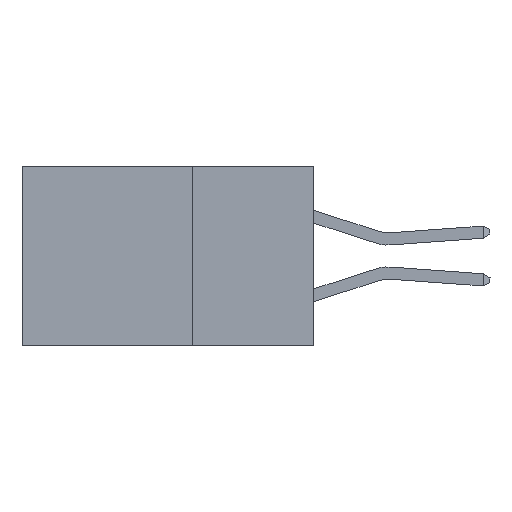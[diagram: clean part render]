
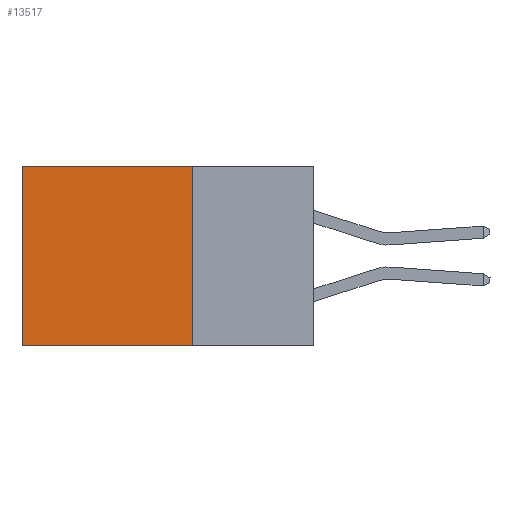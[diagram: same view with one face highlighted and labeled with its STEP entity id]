
A CAD part, left-side view. The second image highlights one B-rep face of the part: STEP entity #13517.
In plain terms, the highlighted planar face has unit normal (-1, 0, 0).
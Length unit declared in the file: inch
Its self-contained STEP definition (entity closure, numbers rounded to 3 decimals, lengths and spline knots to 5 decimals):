
#1093 = AXIS2_PLACEMENT_3D ( 'NONE', #13109, #39738, #36252 ) ;
#1731 = VERTEX_POINT ( 'NONE', #4457 ) ;
#2899 = PLANE ( 'NONE',  #1093 ) ;
#4457 = CARTESIAN_POINT ( 'NONE',  ( 0.2875, 0.25, 0. ) ) ;
#6165 = VERTEX_POINT ( 'NONE', #38595 ) ;
#7071 = ORIENTED_EDGE ( 'NONE', *, *, #35194, .F. ) ;
#8309 = ORIENTED_EDGE ( 'NONE', *, *, #19649, .T. ) ;
#9056 = VECTOR ( 'NONE', #27828, 39.37008 ) ;
#9360 = VERTEX_POINT ( 'NONE', #19835 ) ;
#10572 = CARTESIAN_POINT ( 'NONE',  ( 0.2875, 0.25, -0.37 ) ) ;
#13109 = CARTESIAN_POINT ( 'NONE',  ( 0.2875, 0.25, 0. ) ) ;
#13501 = EDGE_CURVE ( 'NONE', #6165, #21395, #30585, .T. ) ;
#13517 = ADVANCED_FACE ( 'NONE', ( #21168 ), #2899, .F. ) ;
#15517 = EDGE_CURVE ( 'NONE', #1731, #9360, #16249, .T. ) ;
#16249 = LINE ( 'NONE', #28277, #21497 ) ;
#19649 = EDGE_CURVE ( 'NONE', #1731, #6165, #43074, .T. ) ;
#19835 = CARTESIAN_POINT ( 'NONE',  ( 0.2875, 0.25, -0.37 ) ) ;
#21168 = FACE_OUTER_BOUND ( 'NONE', #21216, .T. ) ;
#21216 = EDGE_LOOP ( 'NONE', ( #24120, #7071, #38172, #8309 ) ) ;
#21395 = VERTEX_POINT ( 'NONE', #33671 ) ;
#21497 = VECTOR ( 'NONE', #24767, 39.37008 ) ;
#24120 = ORIENTED_EDGE ( 'NONE', *, *, #13501, .T. ) ;
#24767 = DIRECTION ( 'NONE',  ( 0., 0., -1. ) ) ;
#25999 = DIRECTION ( 'NONE',  ( 0., 0., -1. ) ) ;
#26293 = LINE ( 'NONE', #10572, #37296 ) ;
#27828 = DIRECTION ( 'NONE',  ( 0., 1., 0. ) ) ;
#28277 = CARTESIAN_POINT ( 'NONE',  ( 0.2875, 0.25, 0. ) ) ;
#30585 = LINE ( 'NONE', #36102, #32677 ) ;
#32677 = VECTOR ( 'NONE', #25999, 39.37008 ) ;
#33671 = CARTESIAN_POINT ( 'NONE',  ( 0.2875, 0.6, -0.37 ) ) ;
#34555 = DIRECTION ( 'NONE',  ( 0., 1., 0. ) ) ;
#35194 = EDGE_CURVE ( 'NONE', #9360, #21395, #26293, .T. ) ;
#36102 = CARTESIAN_POINT ( 'NONE',  ( 0.2875, 0.6, 0. ) ) ;
#36252 = DIRECTION ( 'NONE',  ( 0., 0., -1. ) ) ;
#37296 = VECTOR ( 'NONE', #34555, 39.37008 ) ;
#38172 = ORIENTED_EDGE ( 'NONE', *, *, #15517, .F. ) ;
#38190 = CARTESIAN_POINT ( 'NONE',  ( 0.2875, 0.25, 0. ) ) ;
#38595 = CARTESIAN_POINT ( 'NONE',  ( 0.2875, 0.6, 0. ) ) ;
#39738 = DIRECTION ( 'NONE',  ( 1., 0., 0. ) ) ;
#43074 = LINE ( 'NONE', #38190, #9056 ) ;
